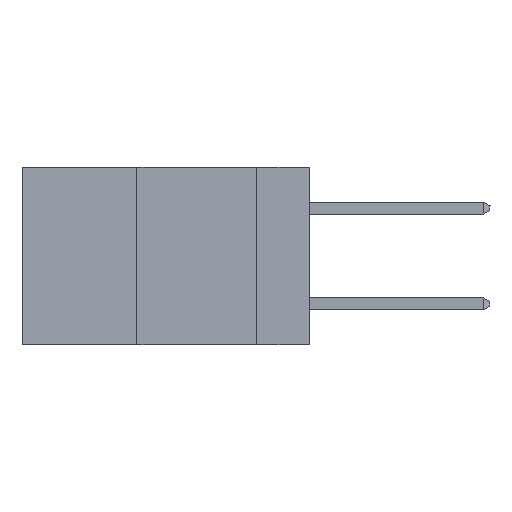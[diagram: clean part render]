
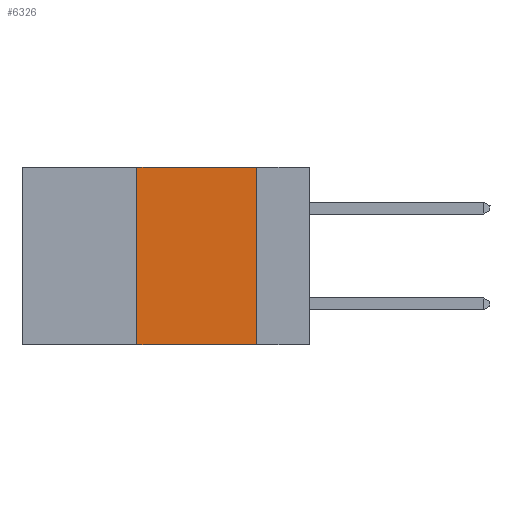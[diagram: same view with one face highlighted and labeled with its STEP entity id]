
A CAD part, left-side view. The second image highlights one B-rep face of the part: STEP entity #6326.
In plain terms, the highlighted planar face has unit normal (-1, 0, 0).
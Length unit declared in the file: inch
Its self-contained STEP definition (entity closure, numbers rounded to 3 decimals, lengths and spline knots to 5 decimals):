
#7 = LINE ( 'NONE', #6433, #6029 ) ;
#1080 = EDGE_CURVE ( 'NONE', #7878, #4107, #7, .T. ) ;
#2321 = LINE ( 'NONE', #10448, #14068 ) ;
#3562 = CARTESIAN_POINT ( 'NONE',  ( 0., 0.36, 0. ) ) ;
#3767 = DIRECTION ( 'NONE',  ( 0., 0., 1. ) ) ;
#4107 = VERTEX_POINT ( 'NONE', #12812 ) ;
#4595 = CARTESIAN_POINT ( 'NONE',  ( 0., 0.36, 0. ) ) ;
#4747 = DIRECTION ( 'NONE',  ( 0., -1., 0. ) ) ;
#5019 = VERTEX_POINT ( 'NONE', #8677 ) ;
#5890 = EDGE_CURVE ( 'NONE', #7878, #14346, #10473, .T. ) ;
#6029 = VECTOR ( 'NONE', #4747, 39.37008 ) ;
#6326 = ADVANCED_FACE ( 'NONE', ( #9762 ), #9142, .F. ) ;
#6433 = CARTESIAN_POINT ( 'NONE',  ( 0., 0.6, -0.37 ) ) ;
#6666 = EDGE_CURVE ( 'NONE', #5019, #4107, #2321, .T. ) ;
#7693 = EDGE_LOOP ( 'NONE', ( #10504, #10531, #10614, #10644 ) ) ;
#7878 = VERTEX_POINT ( 'NONE', #9417 ) ;
#8549 = DIRECTION ( 'NONE',  ( 0., 0., -1. ) ) ;
#8677 = CARTESIAN_POINT ( 'NONE',  ( 0., 0.11, 0. ) ) ;
#8695 = DIRECTION ( 'NONE',  ( 1., 0., 0. ) ) ;
#9055 = CARTESIAN_POINT ( 'NONE',  ( 0., 0.6, 0. ) ) ;
#9142 = PLANE ( 'NONE',  #12578 ) ;
#9417 = CARTESIAN_POINT ( 'NONE',  ( 0., 0.36, -0.37 ) ) ;
#9762 = FACE_OUTER_BOUND ( 'NONE', #7693, .T. ) ;
#10133 = VECTOR ( 'NONE', #3767, 39.37008 ) ;
#10448 = CARTESIAN_POINT ( 'NONE',  ( 0., 0.11, 0. ) ) ;
#10473 = LINE ( 'NONE', #3562, #10133 ) ;
#10504 = ORIENTED_EDGE ( 'NONE', *, *, #6666, .F. ) ;
#10531 = ORIENTED_EDGE ( 'NONE', *, *, #14654, .F. ) ;
#10614 = ORIENTED_EDGE ( 'NONE', *, *, #5890, .F. ) ;
#10644 = ORIENTED_EDGE ( 'NONE', *, *, #1080, .T. ) ;
#10780 = DIRECTION ( 'NONE',  ( 0., -1., 0. ) ) ;
#10947 = DIRECTION ( 'NONE',  ( 0., 0., -1. ) ) ;
#11757 = LINE ( 'NONE', #11908, #13961 ) ;
#11908 = CARTESIAN_POINT ( 'NONE',  ( 0., 0.6, 0. ) ) ;
#12578 = AXIS2_PLACEMENT_3D ( 'NONE', #9055, #8695, #8549 ) ;
#12812 = CARTESIAN_POINT ( 'NONE',  ( 0., 0.11, -0.37 ) ) ;
#13961 = VECTOR ( 'NONE', #10780, 39.37008 ) ;
#14068 = VECTOR ( 'NONE', #10947, 39.37008 ) ;
#14346 = VERTEX_POINT ( 'NONE', #4595 ) ;
#14654 = EDGE_CURVE ( 'NONE', #14346, #5019, #11757, .T. ) ;
